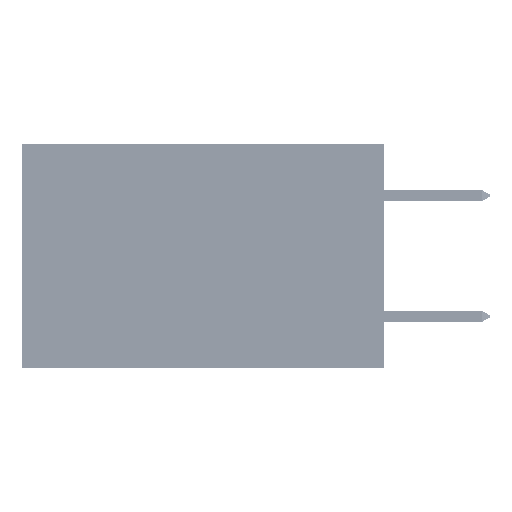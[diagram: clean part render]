
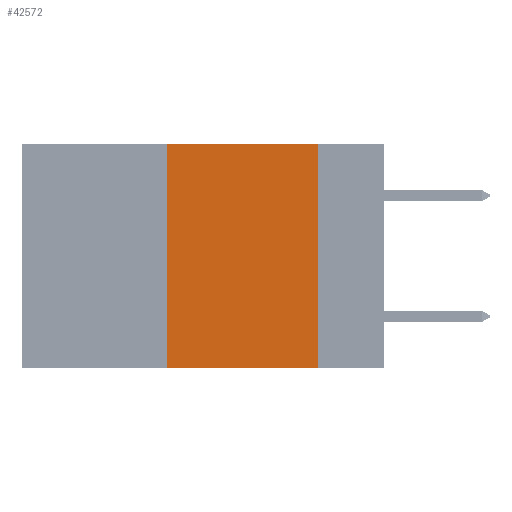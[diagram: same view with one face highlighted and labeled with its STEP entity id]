
A CAD part, left-side view. The second image highlights one B-rep face of the part: STEP entity #42572.
In plain terms, the highlighted planar face has unit normal (-1, 0, 0).
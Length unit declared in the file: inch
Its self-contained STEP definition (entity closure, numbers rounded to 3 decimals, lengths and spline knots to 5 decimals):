
#1059 = CARTESIAN_POINT ( 'NONE',  ( 0., 0.36, 0. ) ) ;
#7913 = CARTESIAN_POINT ( 'NONE',  ( 0., 0.36, -0.37 ) ) ;
#8021 = EDGE_LOOP ( 'NONE', ( #47629, #48354, #8794, #27255 ) ) ;
#8794 = ORIENTED_EDGE ( 'NONE', *, *, #49166, .F. ) ;
#9184 = LINE ( 'NONE', #1059, #47279 ) ;
#13554 = VECTOR ( 'NONE', #51240, 39.37008 ) ;
#14263 = AXIS2_PLACEMENT_3D ( 'NONE', #18401, #39858, #14499 ) ;
#14499 = DIRECTION ( 'NONE',  ( 0., 0., -1. ) ) ;
#14696 = CARTESIAN_POINT ( 'NONE',  ( 0., 0.6, 0. ) ) ;
#15153 = VECTOR ( 'NONE', #29918, 39.37008 ) ;
#16852 = VERTEX_POINT ( 'NONE', #48371 ) ;
#18089 = LINE ( 'NONE', #14696, #47418 ) ;
#18401 = CARTESIAN_POINT ( 'NONE',  ( 0., 0.6, 0. ) ) ;
#24509 = CARTESIAN_POINT ( 'NONE',  ( 0., 0.11, -0.37 ) ) ;
#26541 = PLANE ( 'NONE',  #14263 ) ;
#27255 = ORIENTED_EDGE ( 'NONE', *, *, #43591, .T. ) ;
#27263 = EDGE_CURVE ( 'NONE', #41839, #16852, #18089, .T. ) ;
#27780 = FACE_OUTER_BOUND ( 'NONE', #8021, .T. ) ;
#28454 = VERTEX_POINT ( 'NONE', #24509 ) ;
#29628 = DIRECTION ( 'NONE',  ( 0., -1., 0. ) ) ;
#29918 = DIRECTION ( 'NONE',  ( 0., -1., 0. ) ) ;
#30172 = LINE ( 'NONE', #42282, #15153 ) ;
#30181 = CARTESIAN_POINT ( 'NONE',  ( 0., 0.11, 0. ) ) ;
#32400 = CARTESIAN_POINT ( 'NONE',  ( 0., 0.36, 0. ) ) ;
#38328 = LINE ( 'NONE', #30181, #13554 ) ;
#39382 = VERTEX_POINT ( 'NONE', #7913 ) ;
#39858 = DIRECTION ( 'NONE',  ( 1., 0., 0. ) ) ;
#41839 = VERTEX_POINT ( 'NONE', #32400 ) ;
#42282 = CARTESIAN_POINT ( 'NONE',  ( 0., 0.6, -0.37 ) ) ;
#42572 = ADVANCED_FACE ( 'NONE', ( #27780 ), #26541, .F. ) ;
#43591 = EDGE_CURVE ( 'NONE', #39382, #28454, #30172, .T. ) ;
#44955 = EDGE_CURVE ( 'NONE', #16852, #28454, #38328, .T. ) ;
#47279 = VECTOR ( 'NONE', #48328, 39.37008 ) ;
#47418 = VECTOR ( 'NONE', #29628, 39.37008 ) ;
#47629 = ORIENTED_EDGE ( 'NONE', *, *, #44955, .F. ) ;
#48328 = DIRECTION ( 'NONE',  ( 0., 0., 1. ) ) ;
#48354 = ORIENTED_EDGE ( 'NONE', *, *, #27263, .F. ) ;
#48371 = CARTESIAN_POINT ( 'NONE',  ( 0., 0.11, 0. ) ) ;
#49166 = EDGE_CURVE ( 'NONE', #39382, #41839, #9184, .T. ) ;
#51240 = DIRECTION ( 'NONE',  ( 0., 0., -1. ) ) ;
